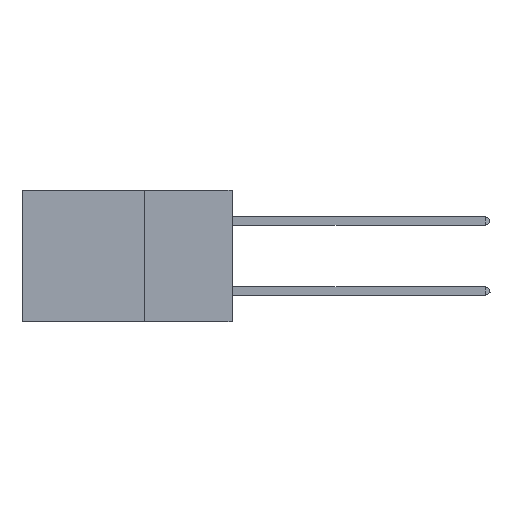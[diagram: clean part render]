
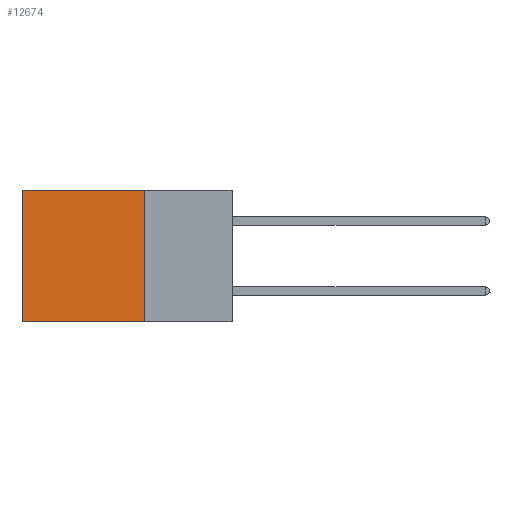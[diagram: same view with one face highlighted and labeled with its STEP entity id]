
A CAD part, left-side view. The second image highlights one B-rep face of the part: STEP entity #12674.
In plain terms, the highlighted planar face has unit normal (-1, 0, 0).
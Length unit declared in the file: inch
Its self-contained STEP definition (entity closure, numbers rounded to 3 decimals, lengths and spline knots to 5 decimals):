
#1416 = CARTESIAN_POINT ( 'NONE',  ( 0.2875, 0.25, -0.375 ) ) ;
#1481 = FACE_OUTER_BOUND ( 'NONE', #15709, .T. ) ;
#3368 = DIRECTION ( 'NONE',  ( 1., 0., 0. ) ) ;
#3380 = VECTOR ( 'NONE', #14793, 39.37008 ) ;
#4099 = EDGE_CURVE ( 'NONE', #17548, #15726, #6941, .T. ) ;
#4360 = AXIS2_PLACEMENT_3D ( 'NONE', #11928, #3368, #13351 ) ;
#4720 = VERTEX_POINT ( 'NONE', #4845 ) ;
#4845 = CARTESIAN_POINT ( 'NONE',  ( 0.2875, 0.6, -0.375 ) ) ;
#4996 = ORIENTED_EDGE ( 'NONE', *, *, #17322, .T. ) ;
#5000 = DIRECTION ( 'NONE',  ( 0., 1., 0. ) ) ;
#5496 = LINE ( 'NONE', #9388, #11344 ) ;
#5749 = EDGE_CURVE ( 'NONE', #18032, #4720, #15823, .T. ) ;
#6262 = DIRECTION ( 'NONE',  ( 0., 1., 0. ) ) ;
#6941 = LINE ( 'NONE', #10518, #17925 ) ;
#7452 = ORIENTED_EDGE ( 'NONE', *, *, #4099, .T. ) ;
#7735 = PLANE ( 'NONE',  #4360 ) ;
#9388 = CARTESIAN_POINT ( 'NONE',  ( 0.2875, 0.6, -0.375 ) ) ;
#9817 = DIRECTION ( 'NONE',  ( 0., 0., -1. ) ) ;
#9897 = LINE ( 'NONE', #13217, #3380 ) ;
#10518 = CARTESIAN_POINT ( 'NONE',  ( 0.2875, 0.25, 0. ) ) ;
#11344 = VECTOR ( 'NONE', #9817, 39.37008 ) ;
#11547 = CARTESIAN_POINT ( 'NONE',  ( 0.2875, 0.6, 0. ) ) ;
#11928 = CARTESIAN_POINT ( 'NONE',  ( 0.2875, 0.25, -0.375 ) ) ;
#12115 = ORIENTED_EDGE ( 'NONE', *, *, #5749, .F. ) ;
#12331 = CARTESIAN_POINT ( 'NONE',  ( 0.2875, 0.25, -0.375 ) ) ;
#12674 = ADVANCED_FACE ( 'NONE', ( #1481 ), #7735, .F. ) ;
#13135 = CARTESIAN_POINT ( 'NONE',  ( 0.2875, 0.25, 0. ) ) ;
#13217 = CARTESIAN_POINT ( 'NONE',  ( 0.2875, 0.25, -0.375 ) ) ;
#13351 = DIRECTION ( 'NONE',  ( 0., 0., -1. ) ) ;
#13733 = ORIENTED_EDGE ( 'NONE', *, *, #13872, .F. ) ;
#13872 = EDGE_CURVE ( 'NONE', #17548, #18032, #9897, .T. ) ;
#14793 = DIRECTION ( 'NONE',  ( 0., 0., -1. ) ) ;
#14940 = VECTOR ( 'NONE', #5000, 39.37008 ) ;
#15709 = EDGE_LOOP ( 'NONE', ( #4996, #12115, #13733, #7452 ) ) ;
#15726 = VERTEX_POINT ( 'NONE', #11547 ) ;
#15823 = LINE ( 'NONE', #12331, #14940 ) ;
#17322 = EDGE_CURVE ( 'NONE', #15726, #4720, #5496, .T. ) ;
#17548 = VERTEX_POINT ( 'NONE', #13135 ) ;
#17925 = VECTOR ( 'NONE', #6262, 39.37008 ) ;
#18032 = VERTEX_POINT ( 'NONE', #1416 ) ;
